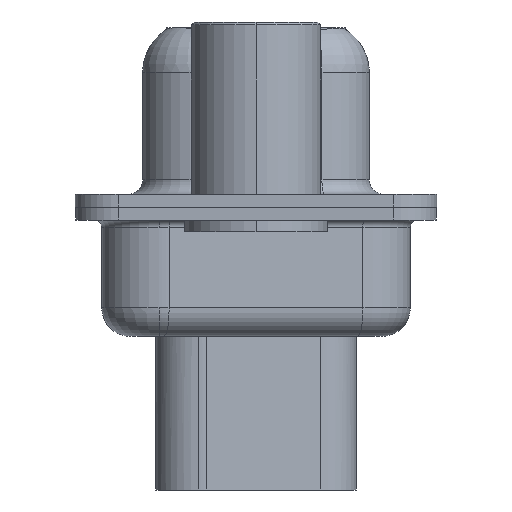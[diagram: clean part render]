
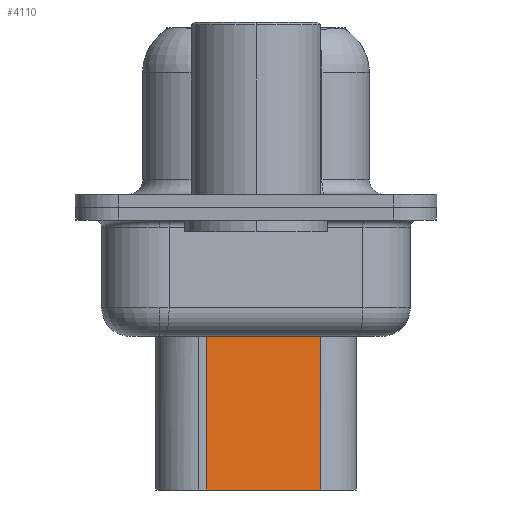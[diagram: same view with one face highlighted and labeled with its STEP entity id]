
A CAD part, left-side view. The second image highlights one B-rep face of the part: STEP entity #4110.
In plain terms, the highlighted planar face has unit normal (-0.985, -0.174, 0).
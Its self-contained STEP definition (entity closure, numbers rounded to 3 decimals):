
#136 = CARTESIAN_POINT ( 'NONE',  ( 4.519, 1.74, -3.1 ) ) ;
#471 = ORIENTED_EDGE ( 'NONE', *, *, #6869, .T. ) ;
#793 = CARTESIAN_POINT ( 'NONE',  ( 5.224, -2.26, -9.85 ) ) ;
#1254 = DIRECTION ( 'NONE',  ( -0.174, 0.985, 0. ) ) ;
#1347 = ORIENTED_EDGE ( 'NONE', *, *, #11355, .F. ) ;
#1508 = CARTESIAN_POINT ( 'NONE',  ( 4.519, 1.74, -9.85 ) ) ;
#1787 = PLANE ( 'NONE',  #11959 ) ;
#1874 = CARTESIAN_POINT ( 'NONE',  ( 5.224, -2.26, -3.975 ) ) ;
#2374 = CARTESIAN_POINT ( 'NONE',  ( 4.519, 1.74, -3.975 ) ) ;
#2536 = CARTESIAN_POINT ( 'NONE',  ( 5.224, -2.26, -3.1 ) ) ;
#2988 = VERTEX_POINT ( 'NONE', #2374 ) ;
#3606 = LINE ( 'NONE', #136, #11893 ) ;
#3718 = LINE ( 'NONE', #1508, #5077 ) ;
#4110 = ADVANCED_FACE ( 'NONE', ( #5334 ), #1787, .T. ) ;
#4287 = VECTOR ( 'NONE', #1254, 1000. ) ;
#4770 = DIRECTION ( 'NONE',  ( 0., 0., -1. ) ) ;
#4885 = DIRECTION ( 'NONE',  ( 0., 0., -1. ) ) ;
#4904 = DIRECTION ( 'NONE',  ( -0.174, 0.985, 0. ) ) ;
#5037 = VERTEX_POINT ( 'NONE', #1874 ) ;
#5077 = VECTOR ( 'NONE', #4904, 1000. ) ;
#5094 = EDGE_CURVE ( 'NONE', #2988, #7127, #3606, .T. ) ;
#5334 = FACE_OUTER_BOUND ( 'NONE', #9100, .T. ) ;
#5927 = EDGE_CURVE ( 'NONE', #14827, #7127, #3718, .T. ) ;
#6581 = CARTESIAN_POINT ( 'NONE',  ( 4.519, 1.74, -3.1 ) ) ;
#6869 = EDGE_CURVE ( 'NONE', #5037, #2988, #13434, .T. ) ;
#7060 = ORIENTED_EDGE ( 'NONE', *, *, #5927, .F. ) ;
#7127 = VERTEX_POINT ( 'NONE', #11300 ) ;
#8317 = CARTESIAN_POINT ( 'NONE',  ( 4.348, 2.709, -3.975 ) ) ;
#8426 = VECTOR ( 'NONE', #4770, 1000. ) ;
#9100 = EDGE_LOOP ( 'NONE', ( #1347, #471, #15200, #7060 ) ) ;
#11300 = CARTESIAN_POINT ( 'NONE',  ( 4.519, 1.74, -9.85 ) ) ;
#11355 = EDGE_CURVE ( 'NONE', #5037, #14827, #14495, .T. ) ;
#11442 = DIRECTION ( 'NONE',  ( 0.174, -0.985, 0. ) ) ;
#11893 = VECTOR ( 'NONE', #4885, 1000. ) ;
#11959 = AXIS2_PLACEMENT_3D ( 'NONE', #6581, #13958, #11442 ) ;
#13434 = LINE ( 'NONE', #8317, #4287 ) ;
#13958 = DIRECTION ( 'NONE',  ( -0.985, -0.174, 0. ) ) ;
#14495 = LINE ( 'NONE', #2536, #8426 ) ;
#14827 = VERTEX_POINT ( 'NONE', #793 ) ;
#15200 = ORIENTED_EDGE ( 'NONE', *, *, #5094, .T. ) ;
